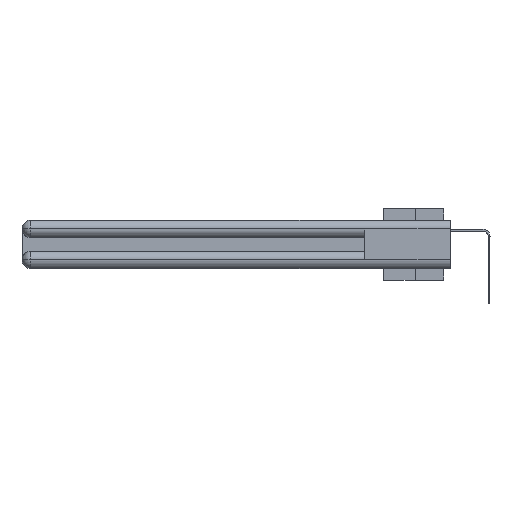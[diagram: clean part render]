
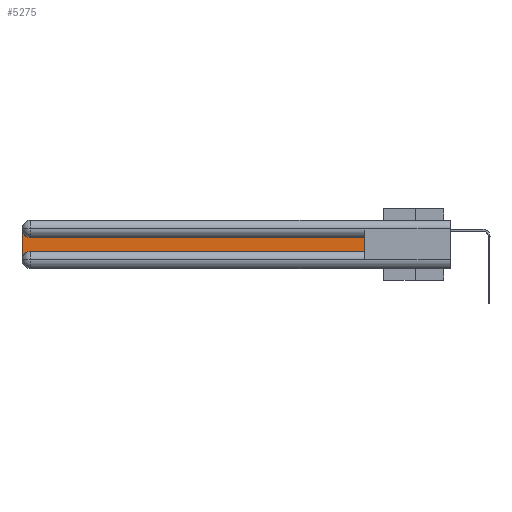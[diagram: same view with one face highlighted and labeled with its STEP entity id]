
A CAD part, left-side view. The second image highlights one B-rep face of the part: STEP entity #5275.
In plain terms, the highlighted planar face has unit normal (-1, 0, 0).
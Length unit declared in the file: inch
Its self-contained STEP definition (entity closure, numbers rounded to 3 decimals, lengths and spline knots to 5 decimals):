
#778 = EDGE_LOOP ( 'NONE', ( #28490, #24739, #36102, #29233, #6094, #4417 ) ) ;
#1715 = DIRECTION ( 'NONE',  ( 0., 0., 1. ) ) ;
#1919 = CARTESIAN_POINT ( 'NONE',  ( 0.075, 0.6, -0.1225 ) ) ;
#1957 = CARTESIAN_POINT ( 'NONE',  ( 0.075, 0.6, -0.2175 ) ) ;
#2037 = CARTESIAN_POINT ( 'NONE',  ( 0.075, 2.94, -0.0625 ) ) ;
#2892 = CARTESIAN_POINT ( 'NONE',  ( 0.075, 2.94, -0.1225 ) ) ;
#3866 = VERTEX_POINT ( 'NONE', #18354 ) ;
#3962 = VECTOR ( 'NONE', #1715, 39.37008 ) ;
#4417 = ORIENTED_EDGE ( 'NONE', *, *, #36763, .T. ) ;
#4622 = DIRECTION ( 'NONE',  ( 0., 0., -1. ) ) ;
#5140 = DIRECTION ( 'NONE',  ( 0., 1., 0. ) ) ;
#5275 = ADVANCED_FACE ( 'NONE', ( #11837 ), #24951, .F. ) ;
#5282 = EDGE_CURVE ( 'NONE', #12818, #3866, #7239, .T. ) ;
#6094 = ORIENTED_EDGE ( 'NONE', *, *, #9382, .T. ) ;
#6651 = CIRCLE ( 'NONE', #26054, 0.06 ) ;
#6758 = VERTEX_POINT ( 'NONE', #9852 ) ;
#7239 = CIRCLE ( 'NONE', #25575, 0.06 ) ;
#8017 = LINE ( 'NONE', #12550, #32776 ) ;
#9231 = VERTEX_POINT ( 'NONE', #22682 ) ;
#9382 = EDGE_CURVE ( 'NONE', #3866, #23972, #20027, .T. ) ;
#9852 = CARTESIAN_POINT ( 'NONE',  ( 0.075, 3., -0.0625 ) ) ;
#9866 = CARTESIAN_POINT ( 'NONE',  ( 0.075, 3., -0.1225 ) ) ;
#10740 = VECTOR ( 'NONE', #5140, 39.37008 ) ;
#11837 = FACE_OUTER_BOUND ( 'NONE', #778, .T. ) ;
#12550 = CARTESIAN_POINT ( 'NONE',  ( 0.075, 3., -0.2175 ) ) ;
#12818 = VERTEX_POINT ( 'NONE', #23493 ) ;
#13177 = DIRECTION ( 'NONE',  ( 0., 0., -1. ) ) ;
#13881 = CARTESIAN_POINT ( 'NONE',  ( 0.075, 0.6, -0.2175 ) ) ;
#16136 = DIRECTION ( 'NONE',  ( 1., 0., 0. ) ) ;
#16207 = LINE ( 'NONE', #1919, #10740 ) ;
#16473 = EDGE_CURVE ( 'NONE', #6758, #12818, #8017, .T. ) ;
#16624 = DIRECTION ( 'NONE',  ( 1., 0., 0. ) ) ;
#16760 = EDGE_CURVE ( 'NONE', #9231, #19714, #16207, .T. ) ;
#18354 = CARTESIAN_POINT ( 'NONE',  ( 0.075, 2.94, -0.2175 ) ) ;
#19099 = VECTOR ( 'NONE', #23691, 39.37008 ) ;
#19578 = DIRECTION ( 'NONE',  ( 0., 0., -1. ) ) ;
#19714 = VERTEX_POINT ( 'NONE', #2892 ) ;
#20027 = LINE ( 'NONE', #20743, #19099 ) ;
#20743 = CARTESIAN_POINT ( 'NONE',  ( 0.075, 0.6, -0.2175 ) ) ;
#22682 = CARTESIAN_POINT ( 'NONE',  ( 0.075, 0.6, -0.1225 ) ) ;
#23493 = CARTESIAN_POINT ( 'NONE',  ( 0.075, 3., -0.2775 ) ) ;
#23691 = DIRECTION ( 'NONE',  ( 0., -1., 0. ) ) ;
#23972 = VERTEX_POINT ( 'NONE', #13881 ) ;
#24739 = ORIENTED_EDGE ( 'NONE', *, *, #37432, .T. ) ;
#24951 = PLANE ( 'NONE',  #31504 ) ;
#25575 = AXIS2_PLACEMENT_3D ( 'NONE', #33459, #16136, #4622 ) ;
#26054 = AXIS2_PLACEMENT_3D ( 'NONE', #2037, #16624, #19578 ) ;
#27353 = LINE ( 'NONE', #1957, #3962 ) ;
#28490 = ORIENTED_EDGE ( 'NONE', *, *, #16760, .T. ) ;
#29233 = ORIENTED_EDGE ( 'NONE', *, *, #5282, .T. ) ;
#29987 = DIRECTION ( 'NONE',  ( 0., 0., -1. ) ) ;
#30621 = DIRECTION ( 'NONE',  ( 1., 0., 0. ) ) ;
#31504 = AXIS2_PLACEMENT_3D ( 'NONE', #9866, #30621, #13177 ) ;
#32776 = VECTOR ( 'NONE', #29987, 39.37008 ) ;
#33459 = CARTESIAN_POINT ( 'NONE',  ( 0.075, 2.94, -0.2775 ) ) ;
#36102 = ORIENTED_EDGE ( 'NONE', *, *, #16473, .T. ) ;
#36763 = EDGE_CURVE ( 'NONE', #23972, #9231, #27353, .T. ) ;
#37432 = EDGE_CURVE ( 'NONE', #19714, #6758, #6651, .T. ) ;
